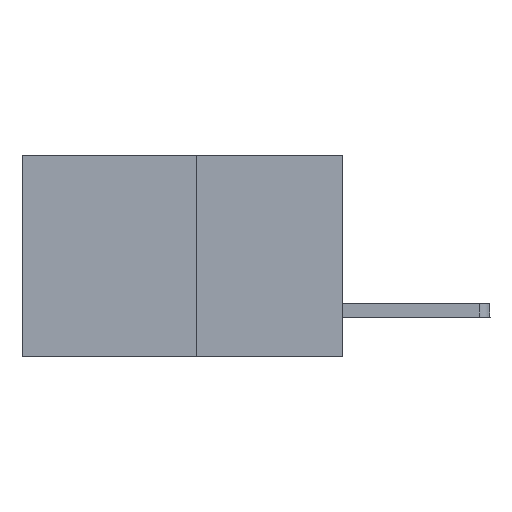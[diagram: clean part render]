
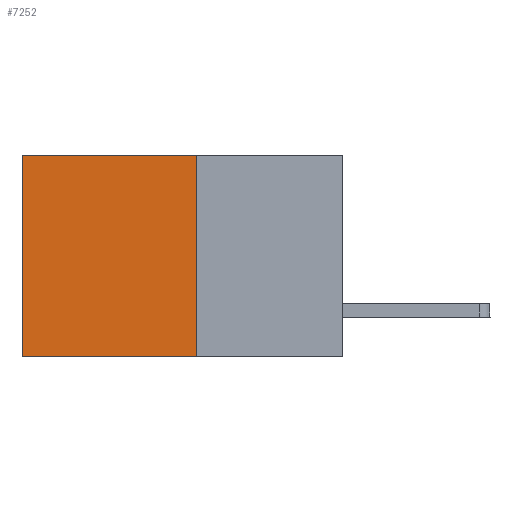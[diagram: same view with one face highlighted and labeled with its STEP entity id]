
A CAD part, left-side view. The second image highlights one B-rep face of the part: STEP entity #7252.
In plain terms, the highlighted planar face has unit normal (-1, 0, 0).
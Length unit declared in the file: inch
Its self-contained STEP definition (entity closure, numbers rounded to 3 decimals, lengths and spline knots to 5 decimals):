
#422 = LINE ( 'NONE', #6717, #3303 ) ;
#474 = ORIENTED_EDGE ( 'NONE', *, *, #2814, .T. ) ;
#574 = DIRECTION ( 'NONE',  ( 0., 1., 0. ) ) ;
#613 = VERTEX_POINT ( 'NONE', #3926 ) ;
#638 = CARTESIAN_POINT ( 'NONE',  ( 0.277, 0.27, -0.37 ) ) ;
#898 = DIRECTION ( 'NONE',  ( 0., 0., -1. ) ) ;
#965 = EDGE_CURVE ( 'NONE', #8803, #1880, #3861, .T. ) ;
#1575 = EDGE_LOOP ( 'NONE', ( #3508, #6511, #2649, #474 ) ) ;
#1880 = VERTEX_POINT ( 'NONE', #3619 ) ;
#2141 = CARTESIAN_POINT ( 'NONE',  ( 0.277, 0.59, -0.37 ) ) ;
#2458 = DIRECTION ( 'NONE',  ( 1., 0., 0. ) ) ;
#2612 = VECTOR ( 'NONE', #6836, 39.37008 ) ;
#2649 = ORIENTED_EDGE ( 'NONE', *, *, #5029, .F. ) ;
#2814 = EDGE_CURVE ( 'NONE', #613, #8803, #422, .T. ) ;
#3303 = VECTOR ( 'NONE', #574, 39.37008 ) ;
#3347 = AXIS2_PLACEMENT_3D ( 'NONE', #3969, #2458, #898 ) ;
#3508 = ORIENTED_EDGE ( 'NONE', *, *, #965, .T. ) ;
#3619 = CARTESIAN_POINT ( 'NONE',  ( 0.277, 0.59, -0.37 ) ) ;
#3630 = EDGE_CURVE ( 'NONE', #8517, #1880, #4593, .T. ) ;
#3861 = LINE ( 'NONE', #2141, #4887 ) ;
#3926 = CARTESIAN_POINT ( 'NONE',  ( 0.277, 0.27, 0. ) ) ;
#3969 = CARTESIAN_POINT ( 'NONE',  ( 0.277, 0.27, -0.37 ) ) ;
#4593 = LINE ( 'NONE', #5951, #6416 ) ;
#4887 = VECTOR ( 'NONE', #6106, 39.37008 ) ;
#4898 = PLANE ( 'NONE',  #3347 ) ;
#5029 = EDGE_CURVE ( 'NONE', #613, #8517, #10021, .T. ) ;
#5951 = CARTESIAN_POINT ( 'NONE',  ( 0.277, 0.27, -0.37 ) ) ;
#6106 = DIRECTION ( 'NONE',  ( 0., 0., -1. ) ) ;
#6108 = DIRECTION ( 'NONE',  ( 0., 1., 0. ) ) ;
#6166 = CARTESIAN_POINT ( 'NONE',  ( 0.277, 0.59, 0. ) ) ;
#6335 = CARTESIAN_POINT ( 'NONE',  ( 0.277, 0.27, -0.37 ) ) ;
#6416 = VECTOR ( 'NONE', #6108, 39.37008 ) ;
#6511 = ORIENTED_EDGE ( 'NONE', *, *, #3630, .F. ) ;
#6717 = CARTESIAN_POINT ( 'NONE',  ( 0.277, 0.27, 0. ) ) ;
#6836 = DIRECTION ( 'NONE',  ( 0., 0., -1. ) ) ;
#7252 = ADVANCED_FACE ( 'NONE', ( #8869 ), #4898, .F. ) ;
#8517 = VERTEX_POINT ( 'NONE', #6335 ) ;
#8803 = VERTEX_POINT ( 'NONE', #6166 ) ;
#8869 = FACE_OUTER_BOUND ( 'NONE', #1575, .T. ) ;
#10021 = LINE ( 'NONE', #638, #2612 ) ;
